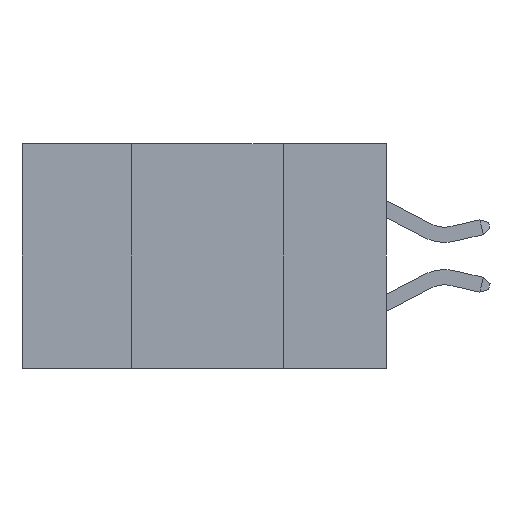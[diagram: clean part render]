
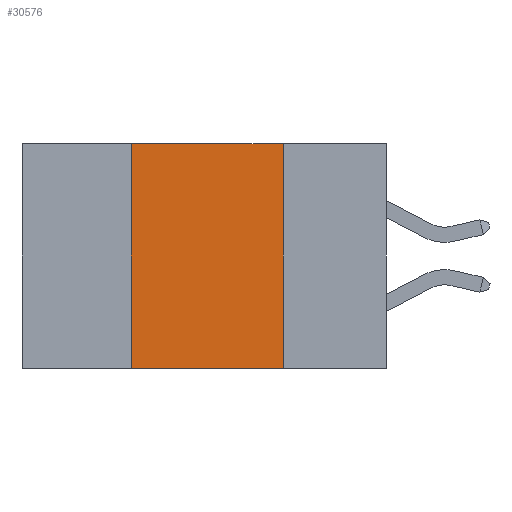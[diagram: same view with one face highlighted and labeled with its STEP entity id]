
A CAD part, left-side view. The second image highlights one B-rep face of the part: STEP entity #30576.
In plain terms, the highlighted planar face has unit normal (-1, 0, 0).
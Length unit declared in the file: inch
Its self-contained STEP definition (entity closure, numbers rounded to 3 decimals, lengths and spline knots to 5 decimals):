
#595 = PLANE ( 'NONE',  #11958 ) ;
#1939 = LINE ( 'NONE', #6519, #7799 ) ;
#2829 = ORIENTED_EDGE ( 'NONE', *, *, #24170, .F. ) ;
#4056 = ORIENTED_EDGE ( 'NONE', *, *, #13994, .F. ) ;
#4351 = VERTEX_POINT ( 'NONE', #7645 ) ;
#6114 = CARTESIAN_POINT ( 'NONE',  ( 0., 0.6, -0.37 ) ) ;
#6519 = CARTESIAN_POINT ( 'NONE',  ( 0., 0.17, 0. ) ) ;
#7645 = CARTESIAN_POINT ( 'NONE',  ( 0., 0.42, -0.37 ) ) ;
#7799 = VECTOR ( 'NONE', #25322, 39.37008 ) ;
#9013 = CARTESIAN_POINT ( 'NONE',  ( 0., 0.6, 0. ) ) ;
#9360 = DIRECTION ( 'NONE',  ( 0., -1., 0. ) ) ;
#10251 = FACE_OUTER_BOUND ( 'NONE', #12377, .T. ) ;
#11958 = AXIS2_PLACEMENT_3D ( 'NONE', #9013, #19459, #25214 ) ;
#12174 = EDGE_CURVE ( 'NONE', #4351, #18339, #24000, .T. ) ;
#12377 = EDGE_LOOP ( 'NONE', ( #2829, #4056, #23603, #20417 ) ) ;
#12505 = CARTESIAN_POINT ( 'NONE',  ( 0., 0.6, 0. ) ) ;
#12594 = LINE ( 'NONE', #12505, #33218 ) ;
#13215 = VERTEX_POINT ( 'NONE', #25145 ) ;
#13994 = EDGE_CURVE ( 'NONE', #18339, #30720, #12594, .T. ) ;
#14116 = CARTESIAN_POINT ( 'NONE',  ( 0., 0.42, 0. ) ) ;
#15592 = EDGE_CURVE ( 'NONE', #4351, #13215, #22138, .T. ) ;
#17082 = CARTESIAN_POINT ( 'NONE',  ( 0., 0.17, 0. ) ) ;
#18339 = VERTEX_POINT ( 'NONE', #14116 ) ;
#18992 = VECTOR ( 'NONE', #33653, 39.37008 ) ;
#19459 = DIRECTION ( 'NONE',  ( 1., 0., 0. ) ) ;
#20417 = ORIENTED_EDGE ( 'NONE', *, *, #15592, .T. ) ;
#22138 = LINE ( 'NONE', #6114, #29731 ) ;
#23603 = ORIENTED_EDGE ( 'NONE', *, *, #12174, .F. ) ;
#24000 = LINE ( 'NONE', #30967, #18992 ) ;
#24170 = EDGE_CURVE ( 'NONE', #30720, #13215, #1939, .T. ) ;
#25145 = CARTESIAN_POINT ( 'NONE',  ( 0., 0.17, -0.37 ) ) ;
#25214 = DIRECTION ( 'NONE',  ( 0., 0., -1. ) ) ;
#25322 = DIRECTION ( 'NONE',  ( 0., 0., -1. ) ) ;
#28064 = DIRECTION ( 'NONE',  ( 0., -1., 0. ) ) ;
#29731 = VECTOR ( 'NONE', #28064, 39.37008 ) ;
#30576 = ADVANCED_FACE ( 'NONE', ( #10251 ), #595, .F. ) ;
#30720 = VERTEX_POINT ( 'NONE', #17082 ) ;
#30967 = CARTESIAN_POINT ( 'NONE',  ( 0., 0.42, 0. ) ) ;
#33218 = VECTOR ( 'NONE', #9360, 39.37008 ) ;
#33653 = DIRECTION ( 'NONE',  ( 0., 0., 1. ) ) ;
